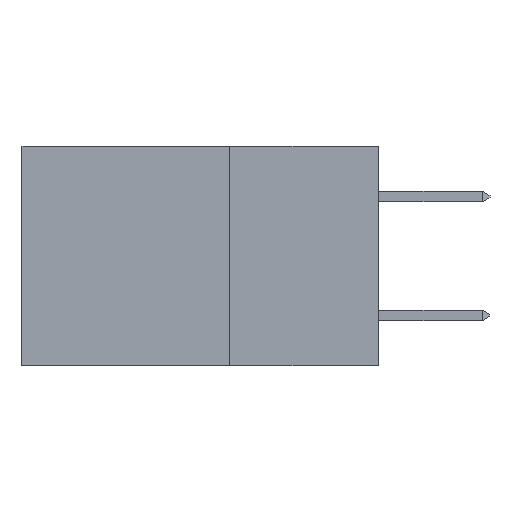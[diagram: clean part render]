
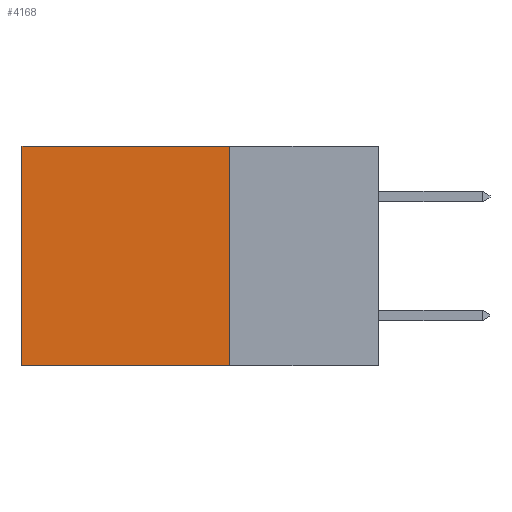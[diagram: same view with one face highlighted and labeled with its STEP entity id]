
A CAD part, left-side view. The second image highlights one B-rep face of the part: STEP entity #4168.
In plain terms, the highlighted planar face has unit normal (-1, 0, 0).
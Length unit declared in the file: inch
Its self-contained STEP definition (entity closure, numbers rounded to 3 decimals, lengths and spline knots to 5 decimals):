
#675 = DIRECTION ( 'NONE',  ( 0., 1., 0. ) ) ;
#788 = VERTEX_POINT ( 'NONE', #19350 ) ;
#1100 = AXIS2_PLACEMENT_3D ( 'NONE', #18811, #18704, #18607 ) ;
#1123 = CARTESIAN_POINT ( 'NONE',  ( 0.298, 0.25, 0. ) ) ;
#1315 = EDGE_CURVE ( 'NONE', #7057, #9859, #6860, .T. ) ;
#1823 = EDGE_CURVE ( 'NONE', #788, #20433, #9718, .T. ) ;
#2588 = CARTESIAN_POINT ( 'NONE',  ( 0.298, 0.25, 0. ) ) ;
#4168 = ADVANCED_FACE ( 'NONE', ( #14670 ), #12036, .F. ) ;
#5207 = ORIENTED_EDGE ( 'NONE', *, *, #10897, .F. ) ;
#6393 = DIRECTION ( 'NONE',  ( 0., 0., -1. ) ) ;
#6860 = LINE ( 'NONE', #1123, #11362 ) ;
#7008 = VECTOR ( 'NONE', #9683, 39.37008 ) ;
#7057 = VERTEX_POINT ( 'NONE', #2588 ) ;
#7352 = ORIENTED_EDGE ( 'NONE', *, *, #1823, .F. ) ;
#8540 = EDGE_LOOP ( 'NONE', ( #14345, #7352, #5207, #11522 ) ) ;
#9683 = DIRECTION ( 'NONE',  ( 0., 0., -1. ) ) ;
#9718 = LINE ( 'NONE', #19453, #13725 ) ;
#9859 = VERTEX_POINT ( 'NONE', #15409 ) ;
#10532 = VECTOR ( 'NONE', #6393, 39.37008 ) ;
#10897 = EDGE_CURVE ( 'NONE', #7057, #788, #11049, .T. ) ;
#11049 = LINE ( 'NONE', #21833, #10532 ) ;
#11362 = VECTOR ( 'NONE', #675, 39.37008 ) ;
#11513 = LINE ( 'NONE', #21760, #7008 ) ;
#11522 = ORIENTED_EDGE ( 'NONE', *, *, #1315, .T. ) ;
#12036 = PLANE ( 'NONE',  #1100 ) ;
#13250 = EDGE_CURVE ( 'NONE', #9859, #20433, #11513, .T. ) ;
#13725 = VECTOR ( 'NONE', #17108, 39.37008 ) ;
#14345 = ORIENTED_EDGE ( 'NONE', *, *, #13250, .T. ) ;
#14670 = FACE_OUTER_BOUND ( 'NONE', #8540, .T. ) ;
#15409 = CARTESIAN_POINT ( 'NONE',  ( 0.298, 0.6, 0. ) ) ;
#17108 = DIRECTION ( 'NONE',  ( 0., 1., 0. ) ) ;
#18607 = DIRECTION ( 'NONE',  ( 0., 0., -1. ) ) ;
#18704 = DIRECTION ( 'NONE',  ( 1., 0., 0. ) ) ;
#18811 = CARTESIAN_POINT ( 'NONE',  ( 0.298, 0.25, 0. ) ) ;
#19284 = CARTESIAN_POINT ( 'NONE',  ( 0.298, 0.6, -0.37 ) ) ;
#19350 = CARTESIAN_POINT ( 'NONE',  ( 0.298, 0.25, -0.37 ) ) ;
#19453 = CARTESIAN_POINT ( 'NONE',  ( 0.298, 0.25, -0.37 ) ) ;
#20433 = VERTEX_POINT ( 'NONE', #19284 ) ;
#21760 = CARTESIAN_POINT ( 'NONE',  ( 0.298, 0.6, 0. ) ) ;
#21833 = CARTESIAN_POINT ( 'NONE',  ( 0.298, 0.25, 0. ) ) ;
